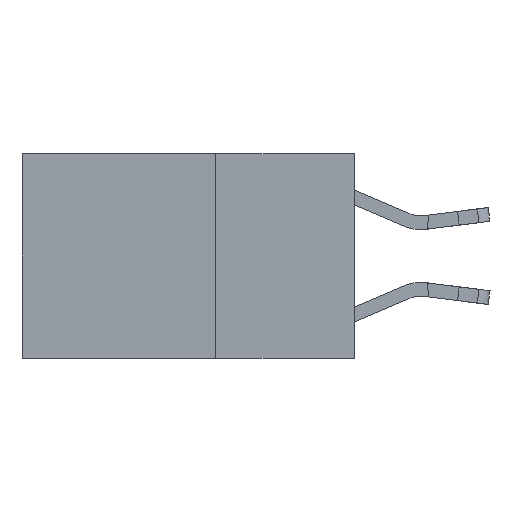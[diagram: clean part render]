
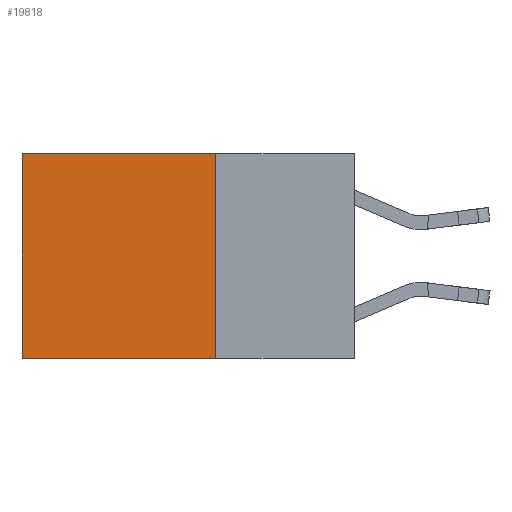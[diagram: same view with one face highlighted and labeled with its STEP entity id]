
A CAD part, left-side view. The second image highlights one B-rep face of the part: STEP entity #19818.
In plain terms, the highlighted planar face has unit normal (-1, 0, 0).
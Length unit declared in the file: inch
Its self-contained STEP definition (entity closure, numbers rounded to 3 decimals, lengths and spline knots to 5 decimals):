
#30 = LINE ( 'NONE', #17485, #17546 ) ;
#2724 = AXIS2_PLACEMENT_3D ( 'NONE', #15104, #21699, #8619 ) ;
#2947 = EDGE_CURVE ( 'NONE', #25720, #20725, #11289, .T. ) ;
#3258 = EDGE_LOOP ( 'NONE', ( #5783, #13439, #25225, #7319 ) ) ;
#3443 = DIRECTION ( 'NONE',  ( 0., 0., -1. ) ) ;
#4057 = CARTESIAN_POINT ( 'NONE',  ( 0.2625, 0.6, 0. ) ) ;
#5783 = ORIENTED_EDGE ( 'NONE', *, *, #2947, .T. ) ;
#7045 = CARTESIAN_POINT ( 'NONE',  ( 0.2625, 0.6, -0.37 ) ) ;
#7319 = ORIENTED_EDGE ( 'NONE', *, *, #7734, .T. ) ;
#7734 = EDGE_CURVE ( 'NONE', #25265, #25720, #13296, .T. ) ;
#8619 = DIRECTION ( 'NONE',  ( 0., 0., -1. ) ) ;
#9087 = VECTOR ( 'NONE', #22040, 39.37008 ) ;
#11008 = EDGE_CURVE ( 'NONE', #25265, #27617, #30, .T. ) ;
#11289 = LINE ( 'NONE', #14339, #16376 ) ;
#12606 = VECTOR ( 'NONE', #18432, 39.37008 ) ;
#13108 = EDGE_CURVE ( 'NONE', #27617, #20725, #20704, .T. ) ;
#13296 = LINE ( 'NONE', #24880, #12606 ) ;
#13439 = ORIENTED_EDGE ( 'NONE', *, *, #13108, .F. ) ;
#14339 = CARTESIAN_POINT ( 'NONE',  ( 0.2625, 0.6, 0. ) ) ;
#15104 = CARTESIAN_POINT ( 'NONE',  ( 0.2625, 0.25, 0. ) ) ;
#16376 = VECTOR ( 'NONE', #3443, 39.37008 ) ;
#16860 = CARTESIAN_POINT ( 'NONE',  ( 0.2625, 0.25, 0. ) ) ;
#17066 = CARTESIAN_POINT ( 'NONE',  ( 0.2625, 0.25, -0.37 ) ) ;
#17485 = CARTESIAN_POINT ( 'NONE',  ( 0.2625, 0.25, 0. ) ) ;
#17546 = VECTOR ( 'NONE', #26834, 39.37008 ) ;
#18432 = DIRECTION ( 'NONE',  ( 0., 1., 0. ) ) ;
#19525 = PLANE ( 'NONE',  #2724 ) ;
#19818 = ADVANCED_FACE ( 'NONE', ( #25620 ), #19525, .F. ) ;
#19860 = CARTESIAN_POINT ( 'NONE',  ( 0.2625, 0.25, -0.37 ) ) ;
#20704 = LINE ( 'NONE', #19860, #9087 ) ;
#20725 = VERTEX_POINT ( 'NONE', #7045 ) ;
#21699 = DIRECTION ( 'NONE',  ( 1., 0., 0. ) ) ;
#22040 = DIRECTION ( 'NONE',  ( 0., 1., 0. ) ) ;
#24880 = CARTESIAN_POINT ( 'NONE',  ( 0.2625, 0.25, 0. ) ) ;
#25225 = ORIENTED_EDGE ( 'NONE', *, *, #11008, .F. ) ;
#25265 = VERTEX_POINT ( 'NONE', #16860 ) ;
#25620 = FACE_OUTER_BOUND ( 'NONE', #3258, .T. ) ;
#25720 = VERTEX_POINT ( 'NONE', #4057 ) ;
#26834 = DIRECTION ( 'NONE',  ( 0., 0., -1. ) ) ;
#27617 = VERTEX_POINT ( 'NONE', #17066 ) ;
